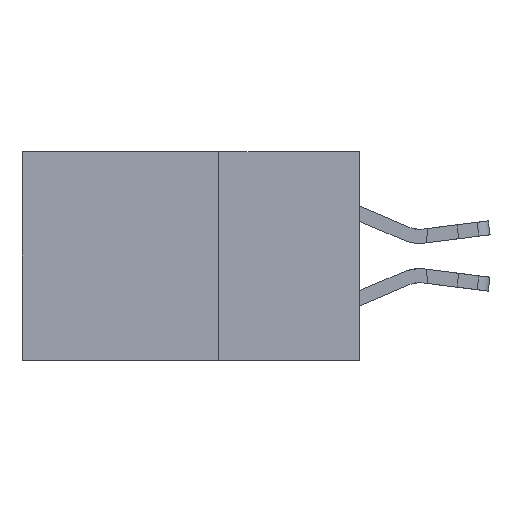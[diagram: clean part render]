
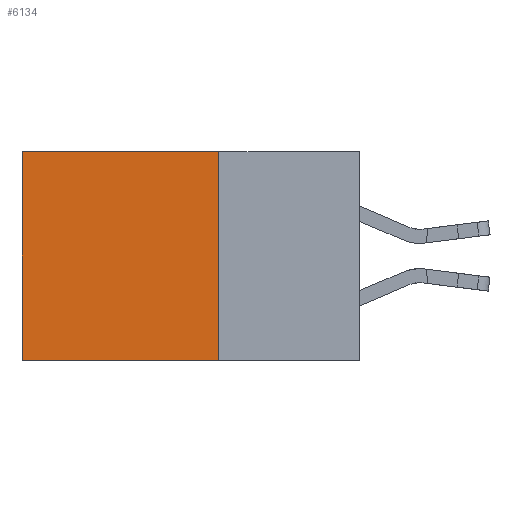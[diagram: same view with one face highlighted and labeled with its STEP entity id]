
A CAD part, left-side view. The second image highlights one B-rep face of the part: STEP entity #6134.
In plain terms, the highlighted planar face has unit normal (-1, 0, 0).
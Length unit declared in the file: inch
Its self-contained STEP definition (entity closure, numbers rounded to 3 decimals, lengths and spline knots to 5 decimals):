
#214 = EDGE_CURVE ( 'NONE', #3136, #23503, #7772, .T. ) ;
#321 = DIRECTION ( 'NONE',  ( 0., 0., -1. ) ) ;
#1894 = VECTOR ( 'NONE', #12692, 39.37008 ) ;
#2272 = CARTESIAN_POINT ( 'NONE',  ( 0.2875, 0.25, 0. ) ) ;
#2666 = LINE ( 'NONE', #7974, #12188 ) ;
#2877 = CARTESIAN_POINT ( 'NONE',  ( 0.2875, 0.25, 0. ) ) ;
#3136 = VERTEX_POINT ( 'NONE', #30212 ) ;
#3175 = AXIS2_PLACEMENT_3D ( 'NONE', #24248, #11261, #31909 ) ;
#3519 = LINE ( 'NONE', #2877, #5843 ) ;
#5310 = ORIENTED_EDGE ( 'NONE', *, *, #214, .F. ) ;
#5843 = VECTOR ( 'NONE', #321, 39.37008 ) ;
#6134 = ADVANCED_FACE ( 'NONE', ( #29175 ), #11090, .F. ) ;
#7539 = ORIENTED_EDGE ( 'NONE', *, *, #21728, .T. ) ;
#7635 = DIRECTION ( 'NONE',  ( 0., 0., -1. ) ) ;
#7772 = LINE ( 'NONE', #31473, #12427 ) ;
#7974 = CARTESIAN_POINT ( 'NONE',  ( 0.2875, 0.6, 0. ) ) ;
#8044 = CARTESIAN_POINT ( 'NONE',  ( 0.2875, 0.6, -0.37 ) ) ;
#11090 = PLANE ( 'NONE',  #3175 ) ;
#11261 = DIRECTION ( 'NONE',  ( 1., 0., 0. ) ) ;
#12188 = VECTOR ( 'NONE', #7635, 39.37008 ) ;
#12427 = VECTOR ( 'NONE', #18527, 39.37008 ) ;
#12692 = DIRECTION ( 'NONE',  ( 0., 1., 0. ) ) ;
#15253 = LINE ( 'NONE', #2272, #1894 ) ;
#15712 = EDGE_CURVE ( 'NONE', #21409, #23503, #2666, .T. ) ;
#16215 = CARTESIAN_POINT ( 'NONE',  ( 0.2875, 0.25, 0. ) ) ;
#18527 = DIRECTION ( 'NONE',  ( 0., 1., 0. ) ) ;
#19061 = ORIENTED_EDGE ( 'NONE', *, *, #24838, .F. ) ;
#21409 = VERTEX_POINT ( 'NONE', #29428 ) ;
#21728 = EDGE_CURVE ( 'NONE', #26049, #21409, #15253, .T. ) ;
#23503 = VERTEX_POINT ( 'NONE', #8044 ) ;
#24248 = CARTESIAN_POINT ( 'NONE',  ( 0.2875, 0.25, 0. ) ) ;
#24838 = EDGE_CURVE ( 'NONE', #26049, #3136, #3519, .T. ) ;
#26049 = VERTEX_POINT ( 'NONE', #16215 ) ;
#28402 = ORIENTED_EDGE ( 'NONE', *, *, #15712, .T. ) ;
#29175 = FACE_OUTER_BOUND ( 'NONE', #30478, .T. ) ;
#29428 = CARTESIAN_POINT ( 'NONE',  ( 0.2875, 0.6, 0. ) ) ;
#30212 = CARTESIAN_POINT ( 'NONE',  ( 0.2875, 0.25, -0.37 ) ) ;
#30478 = EDGE_LOOP ( 'NONE', ( #28402, #5310, #19061, #7539 ) ) ;
#31473 = CARTESIAN_POINT ( 'NONE',  ( 0.2875, 0.25, -0.37 ) ) ;
#31909 = DIRECTION ( 'NONE',  ( 0., 0., -1. ) ) ;
